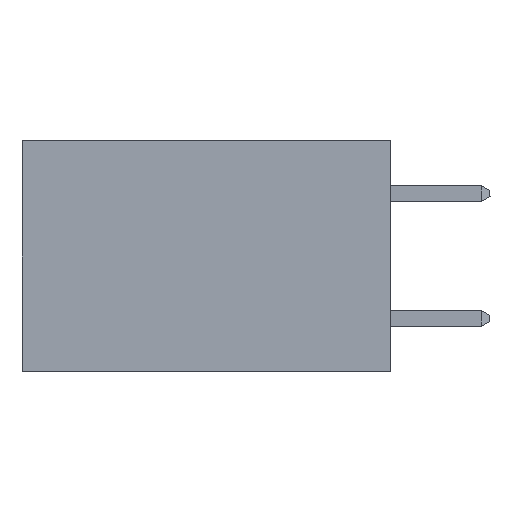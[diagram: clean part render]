
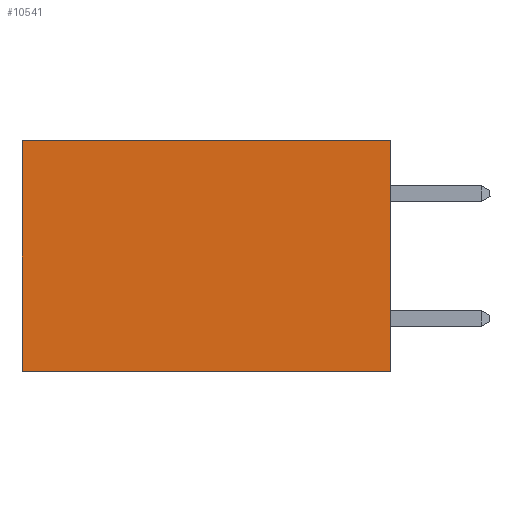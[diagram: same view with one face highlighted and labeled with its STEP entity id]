
A CAD part, left-side view. The second image highlights one B-rep face of the part: STEP entity #10541.
In plain terms, the highlighted planar face has unit normal (-1, 0, 0).
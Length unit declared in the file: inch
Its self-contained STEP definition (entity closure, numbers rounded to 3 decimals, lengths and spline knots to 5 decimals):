
#772 = DIRECTION ( 'NONE',  ( 0., 1., 0. ) ) ;
#1105 = LINE ( 'NONE', #3654, #15970 ) ;
#1206 = CARTESIAN_POINT ( 'NONE',  ( 0.277, 0., 0. ) ) ;
#1831 = VERTEX_POINT ( 'NONE', #6637 ) ;
#2634 = EDGE_CURVE ( 'NONE', #2886, #1831, #1105, .T. ) ;
#2886 = VERTEX_POINT ( 'NONE', #22101 ) ;
#3136 = AXIS2_PLACEMENT_3D ( 'NONE', #4492, #19803, #8373 ) ;
#3498 = EDGE_LOOP ( 'NONE', ( #6693, #9426, #23141, #21060 ) ) ;
#3509 = DIRECTION ( 'NONE',  ( 0., 0., -1. ) ) ;
#3586 = DIRECTION ( 'NONE',  ( 0., 1., 0. ) ) ;
#3654 = CARTESIAN_POINT ( 'NONE',  ( 0.277, 0., -0.37 ) ) ;
#4492 = CARTESIAN_POINT ( 'NONE',  ( 0.277, 0., -0.37 ) ) ;
#4774 = LINE ( 'NONE', #19916, #14495 ) ;
#5502 = VECTOR ( 'NONE', #772, 39.37008 ) ;
#5661 = FACE_OUTER_BOUND ( 'NONE', #3498, .T. ) ;
#6543 = DIRECTION ( 'NONE',  ( 0., 0., -1. ) ) ;
#6637 = CARTESIAN_POINT ( 'NONE',  ( 0.277, 0.59, -0.37 ) ) ;
#6693 = ORIENTED_EDGE ( 'NONE', *, *, #19522, .T. ) ;
#7548 = EDGE_CURVE ( 'NONE', #12680, #9337, #20130, .T. ) ;
#7821 = VECTOR ( 'NONE', #3509, 39.37008 ) ;
#8373 = DIRECTION ( 'NONE',  ( 0., 0., -1. ) ) ;
#8700 = CARTESIAN_POINT ( 'NONE',  ( 0.277, 0.59, 0. ) ) ;
#9074 = LINE ( 'NONE', #18913, #7821 ) ;
#9337 = VERTEX_POINT ( 'NONE', #8700 ) ;
#9426 = ORIENTED_EDGE ( 'NONE', *, *, #2634, .F. ) ;
#9903 = EDGE_CURVE ( 'NONE', #12680, #2886, #4774, .T. ) ;
#10541 = ADVANCED_FACE ( 'NONE', ( #5661 ), #16085, .F. ) ;
#10744 = CARTESIAN_POINT ( 'NONE',  ( 0.277, 0., 0. ) ) ;
#12680 = VERTEX_POINT ( 'NONE', #10744 ) ;
#14495 = VECTOR ( 'NONE', #6543, 39.37008 ) ;
#15970 = VECTOR ( 'NONE', #3586, 39.37008 ) ;
#16085 = PLANE ( 'NONE',  #3136 ) ;
#18913 = CARTESIAN_POINT ( 'NONE',  ( 0.277, 0.59, -0.37 ) ) ;
#19522 = EDGE_CURVE ( 'NONE', #9337, #1831, #9074, .T. ) ;
#19803 = DIRECTION ( 'NONE',  ( 1., 0., 0. ) ) ;
#19916 = CARTESIAN_POINT ( 'NONE',  ( 0.277, 0., -0.37 ) ) ;
#20130 = LINE ( 'NONE', #1206, #5502 ) ;
#21060 = ORIENTED_EDGE ( 'NONE', *, *, #7548, .T. ) ;
#22101 = CARTESIAN_POINT ( 'NONE',  ( 0.277, 0., -0.37 ) ) ;
#23141 = ORIENTED_EDGE ( 'NONE', *, *, #9903, .F. ) ;
